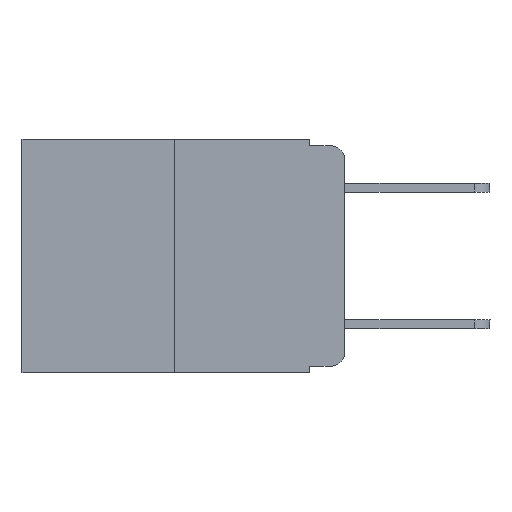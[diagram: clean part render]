
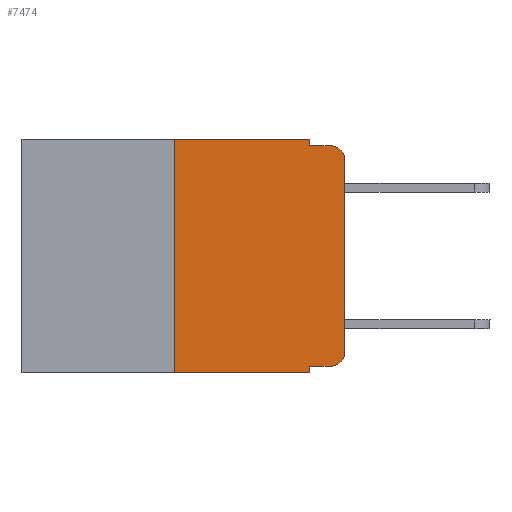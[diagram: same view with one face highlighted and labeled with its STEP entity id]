
A CAD part, left-side view. The second image highlights one B-rep face of the part: STEP entity #7474.
In plain terms, the highlighted planar face has unit normal (-1, 0, 0).
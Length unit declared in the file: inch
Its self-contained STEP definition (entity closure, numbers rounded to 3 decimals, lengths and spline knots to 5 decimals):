
#40 = CARTESIAN_POINT ( 'NONE',  ( 0., 0.051, 0. ) ) ;
#100 = EDGE_CURVE ( 'NONE', #8283, #14322, #3900, .T. ) ;
#527 = DIRECTION ( 'NONE',  ( 0., -1., 0. ) ) ;
#565 = CARTESIAN_POINT ( 'NONE',  ( 0., 0.02, -0.313 ) ) ;
#834 = VECTOR ( 'NONE', #6298, 39.37008 ) ;
#1044 = DIRECTION ( 'NONE',  ( 0., 0., -1. ) ) ;
#1082 = VERTEX_POINT ( 'NONE', #9388 ) ;
#1359 = DIRECTION ( 'NONE',  ( 0., -1., 0. ) ) ;
#1479 = AXIS2_PLACEMENT_3D ( 'NONE', #12415, #6600, #15198 ) ;
#1650 = CARTESIAN_POINT ( 'NONE',  ( 0., 0.051, -0.343 ) ) ;
#1774 = CARTESIAN_POINT ( 'NONE',  ( 0., 0.051, 0. ) ) ;
#1841 = VERTEX_POINT ( 'NONE', #13974 ) ;
#2220 = ORIENTED_EDGE ( 'NONE', *, *, #13558, .F. ) ;
#2327 = DIRECTION ( 'NONE',  ( 0., -1., 0. ) ) ;
#2482 = LINE ( 'NONE', #9863, #15719 ) ;
#2654 = VECTOR ( 'NONE', #8819, 39.37008 ) ;
#2770 = LINE ( 'NONE', #7666, #5226 ) ;
#2824 = LINE ( 'NONE', #5292, #10640 ) ;
#3009 = EDGE_CURVE ( 'NONE', #14322, #7198, #3806, .T. ) ;
#3588 = ORIENTED_EDGE ( 'NONE', *, *, #6680, .F. ) ;
#3688 = EDGE_LOOP ( 'NONE', ( #10906, #11894, #5824, #3588, #2220, #10852, #4221, #5875, #8079, #4724 ) ) ;
#3806 = CIRCLE ( 'NONE', #1479, 0.02 ) ;
#3900 = LINE ( 'NONE', #12496, #2654 ) ;
#4115 = LINE ( 'NONE', #9048, #8435 ) ;
#4221 = ORIENTED_EDGE ( 'NONE', *, *, #9519, .T. ) ;
#4724 = ORIENTED_EDGE ( 'NONE', *, *, #15347, .T. ) ;
#4991 = EDGE_CURVE ( 'NONE', #1082, #7198, #2482, .T. ) ;
#5012 = LINE ( 'NONE', #40, #834 ) ;
#5226 = VECTOR ( 'NONE', #12568, 39.37008 ) ;
#5292 = CARTESIAN_POINT ( 'NONE',  ( 0., 0.473, -0.343 ) ) ;
#5426 = CARTESIAN_POINT ( 'NONE',  ( 0., 0.051, -0.333 ) ) ;
#5467 = DIRECTION ( 'NONE',  ( 0., 0., -1. ) ) ;
#5824 = ORIENTED_EDGE ( 'NONE', *, *, #4991, .F. ) ;
#5875 = ORIENTED_EDGE ( 'NONE', *, *, #13482, .F. ) ;
#5935 = DIRECTION ( 'NONE',  ( 1., 0., 0. ) ) ;
#6298 = DIRECTION ( 'NONE',  ( 0., 0., -1. ) ) ;
#6554 = CARTESIAN_POINT ( 'NONE',  ( 0., 0., -0.03 ) ) ;
#6600 = DIRECTION ( 'NONE',  ( -1., 0., 0. ) ) ;
#6645 = CARTESIAN_POINT ( 'NONE',  ( 0., 0., -0.313 ) ) ;
#6680 = EDGE_CURVE ( 'NONE', #13963, #1082, #5012, .T. ) ;
#6902 = EDGE_CURVE ( 'NONE', #12265, #1841, #2770, .T. ) ;
#6916 = VERTEX_POINT ( 'NONE', #15037 ) ;
#6952 = CARTESIAN_POINT ( 'NONE',  ( 0., 0.02, -0.333 ) ) ;
#7157 = FACE_OUTER_BOUND ( 'NONE', #3688, .T. ) ;
#7198 = VERTEX_POINT ( 'NONE', #8866 ) ;
#7474 = ADVANCED_FACE ( 'NONE', ( #7157 ), #11302, .F. ) ;
#7666 = CARTESIAN_POINT ( 'NONE',  ( 0., 0.25, 0. ) ) ;
#7821 = LINE ( 'NONE', #11592, #10743 ) ;
#8079 = ORIENTED_EDGE ( 'NONE', *, *, #14229, .T. ) ;
#8283 = VERTEX_POINT ( 'NONE', #6645 ) ;
#8358 = CARTESIAN_POINT ( 'NONE',  ( 0., 0.25, -0.343 ) ) ;
#8435 = VECTOR ( 'NONE', #13904, 39.37008 ) ;
#8819 = DIRECTION ( 'NONE',  ( 0., 0., 1. ) ) ;
#8866 = CARTESIAN_POINT ( 'NONE',  ( 0., 0.02, -0.01 ) ) ;
#8905 = CARTESIAN_POINT ( 'NONE',  ( 0., 0.473, 0. ) ) ;
#9048 = CARTESIAN_POINT ( 'NONE',  ( 0., 0.051, 0. ) ) ;
#9388 = CARTESIAN_POINT ( 'NONE',  ( 0., 0.051, -0.01 ) ) ;
#9519 = EDGE_CURVE ( 'NONE', #12265, #11481, #2824, .T. ) ;
#9745 = VECTOR ( 'NONE', #527, 39.37008 ) ;
#9863 = CARTESIAN_POINT ( 'NONE',  ( 0., 0.051, -0.01 ) ) ;
#10322 = DIRECTION ( 'NONE',  ( 0., -1., 0. ) ) ;
#10499 = CIRCLE ( 'NONE', #15351, 0.02 ) ;
#10640 = VECTOR ( 'NONE', #1359, 39.37008 ) ;
#10743 = VECTOR ( 'NONE', #10322, 39.37008 ) ;
#10852 = ORIENTED_EDGE ( 'NONE', *, *, #6902, .F. ) ;
#10906 = ORIENTED_EDGE ( 'NONE', *, *, #100, .T. ) ;
#11302 = PLANE ( 'NONE',  #15492 ) ;
#11481 = VERTEX_POINT ( 'NONE', #1650 ) ;
#11592 = CARTESIAN_POINT ( 'NONE',  ( 0., 0.473, 0. ) ) ;
#11662 = DIRECTION ( 'NONE',  ( -1., 0., 0. ) ) ;
#11894 = ORIENTED_EDGE ( 'NONE', *, *, #3009, .T. ) ;
#12265 = VERTEX_POINT ( 'NONE', #8358 ) ;
#12415 = CARTESIAN_POINT ( 'NONE',  ( 0., 0.02, -0.03 ) ) ;
#12496 = CARTESIAN_POINT ( 'NONE',  ( 0., 0., 0. ) ) ;
#12568 = DIRECTION ( 'NONE',  ( 0., 0., 1. ) ) ;
#13020 = VERTEX_POINT ( 'NONE', #6952 ) ;
#13482 = EDGE_CURVE ( 'NONE', #6916, #11481, #4115, .T. ) ;
#13558 = EDGE_CURVE ( 'NONE', #1841, #13963, #7821, .T. ) ;
#13904 = DIRECTION ( 'NONE',  ( 0., 0., -1. ) ) ;
#13963 = VERTEX_POINT ( 'NONE', #1774 ) ;
#13974 = CARTESIAN_POINT ( 'NONE',  ( 0., 0.25, 0. ) ) ;
#14229 = EDGE_CURVE ( 'NONE', #6916, #13020, #14987, .T. ) ;
#14322 = VERTEX_POINT ( 'NONE', #6554 ) ;
#14987 = LINE ( 'NONE', #5426, #9745 ) ;
#15037 = CARTESIAN_POINT ( 'NONE',  ( 0., 0.051, -0.333 ) ) ;
#15198 = DIRECTION ( 'NONE',  ( 0., 0., -1. ) ) ;
#15347 = EDGE_CURVE ( 'NONE', #13020, #8283, #10499, .T. ) ;
#15351 = AXIS2_PLACEMENT_3D ( 'NONE', #565, #11662, #5467 ) ;
#15492 = AXIS2_PLACEMENT_3D ( 'NONE', #8905, #5935, #1044 ) ;
#15719 = VECTOR ( 'NONE', #2327, 39.37008 ) ;
